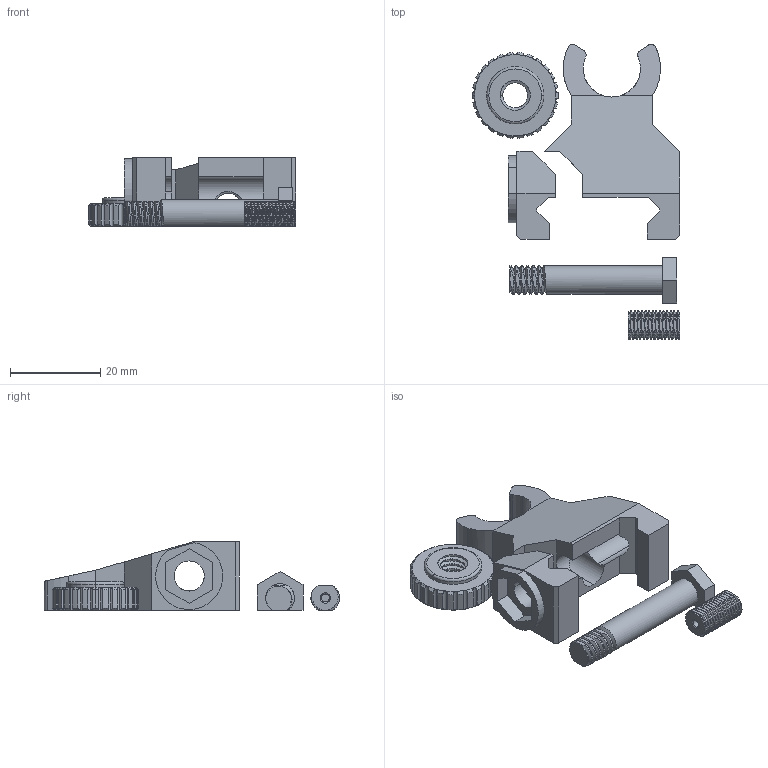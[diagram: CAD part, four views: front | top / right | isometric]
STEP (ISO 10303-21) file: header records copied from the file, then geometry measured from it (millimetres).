
FILE_DESCRIPTION (( 'STEP AP203' ), '1' );
FILE_NAME ('AF-WF-GS-MDL-001-STEP.STEP', '2020-07-21T18:42:15', ( '' ), ( '' ), 'SwSTEP 2.0', 'SolidWorks 2018', '' );
FILE_SCHEMA (( 'CONFIG_CONTROL_DESIGN' ));
Length unit declared in the file: inch
Products named in the file (1): AF-WF-GS-MDL-001-STEP
Bounding box: 46.02 x 65.45 x 15.24 mm (x, y, z)
Volume: 10788.7 mm3; surface area: 7546.7 mm2
Topology: 5 solids, 5 shells, 400 faces, 1053 edges, 669 vertices
Faces by surface type: cylinder 172, plane 128, cone 56, bspline 42, torus 2
Entity records: 33759 total; most frequent: CARTESIAN_POINT 24981, ORIENTED_EDGE 2106, DIRECTION 1480, EDGE_CURVE 1053, VERTEX_POINT 669, AXIS2_PLACEMENT_3D 538, EDGE_LOOP 414, LINE 404
